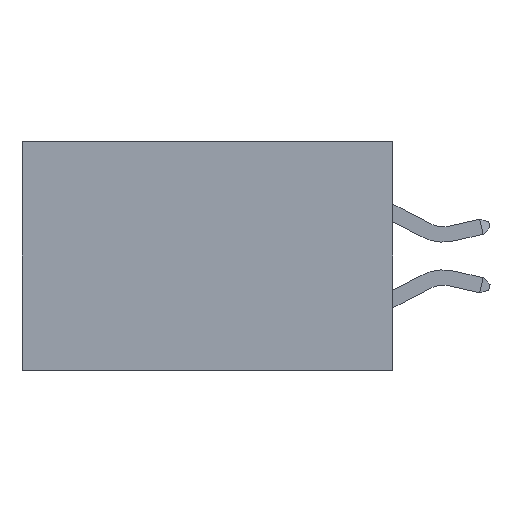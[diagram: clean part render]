
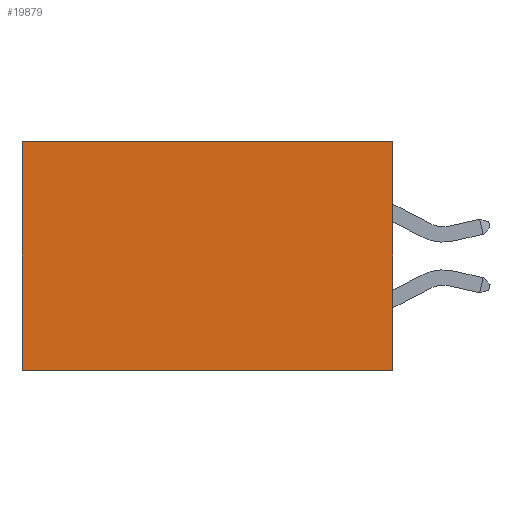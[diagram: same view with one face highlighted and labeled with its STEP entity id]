
A CAD part, left-side view. The second image highlights one B-rep face of the part: STEP entity #19879.
In plain terms, the highlighted planar face has unit normal (-1, 0, 0).
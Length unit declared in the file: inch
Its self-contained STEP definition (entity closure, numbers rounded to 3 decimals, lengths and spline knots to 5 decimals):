
#164 = DIRECTION ( 'NONE',  ( 0., 0., -1. ) ) ;
#1785 = CARTESIAN_POINT ( 'NONE',  ( 0.2875, 0., -0.37 ) ) ;
#3027 = CARTESIAN_POINT ( 'NONE',  ( 0.2875, 0.6, -0.37 ) ) ;
#3044 = CARTESIAN_POINT ( 'NONE',  ( 0.2875, 0., 0. ) ) ;
#3872 = LINE ( 'NONE', #5533, #8000 ) ;
#4692 = EDGE_CURVE ( 'NONE', #20896, #7798, #12696, .T. ) ;
#5347 = ORIENTED_EDGE ( 'NONE', *, *, #21614, .F. ) ;
#5533 = CARTESIAN_POINT ( 'NONE',  ( 0.2875, 0., 0. ) ) ;
#5863 = CARTESIAN_POINT ( 'NONE',  ( 0.2875, 0.6, 0. ) ) ;
#6748 = CARTESIAN_POINT ( 'NONE',  ( 0.2875, 0.6, 0. ) ) ;
#6987 = AXIS2_PLACEMENT_3D ( 'NONE', #3044, #8350, #20275 ) ;
#7798 = VERTEX_POINT ( 'NONE', #5863 ) ;
#8000 = VECTOR ( 'NONE', #164, 39.37008 ) ;
#8153 = CARTESIAN_POINT ( 'NONE',  ( 0.2875, 0., 0. ) ) ;
#8350 = DIRECTION ( 'NONE',  ( 1., 0., 0. ) ) ;
#8469 = DIRECTION ( 'NONE',  ( 0., 0., -1. ) ) ;
#9036 = EDGE_CURVE ( 'NONE', #7798, #14553, #19219, .T. ) ;
#9578 = VECTOR ( 'NONE', #21805, 39.37008 ) ;
#11141 = ORIENTED_EDGE ( 'NONE', *, *, #9036, .T. ) ;
#11676 = CARTESIAN_POINT ( 'NONE',  ( 0.2875, 0., -0.37 ) ) ;
#12696 = LINE ( 'NONE', #16119, #21182 ) ;
#14129 = LINE ( 'NONE', #11676, #9578 ) ;
#14167 = VECTOR ( 'NONE', #8469, 39.37008 ) ;
#14245 = VERTEX_POINT ( 'NONE', #1785 ) ;
#14553 = VERTEX_POINT ( 'NONE', #3027 ) ;
#16114 = FACE_OUTER_BOUND ( 'NONE', #18977, .T. ) ;
#16119 = CARTESIAN_POINT ( 'NONE',  ( 0.2875, 0., 0. ) ) ;
#17276 = ORIENTED_EDGE ( 'NONE', *, *, #21909, .F. ) ;
#18164 = ORIENTED_EDGE ( 'NONE', *, *, #4692, .T. ) ;
#18584 = PLANE ( 'NONE',  #6987 ) ;
#18977 = EDGE_LOOP ( 'NONE', ( #11141, #5347, #17276, #18164 ) ) ;
#19219 = LINE ( 'NONE', #6748, #14167 ) ;
#19456 = DIRECTION ( 'NONE',  ( 0., 1., 0. ) ) ;
#19879 = ADVANCED_FACE ( 'NONE', ( #16114 ), #18584, .F. ) ;
#20275 = DIRECTION ( 'NONE',  ( 0., 0., -1. ) ) ;
#20896 = VERTEX_POINT ( 'NONE', #8153 ) ;
#21182 = VECTOR ( 'NONE', #19456, 39.37008 ) ;
#21614 = EDGE_CURVE ( 'NONE', #14245, #14553, #14129, .T. ) ;
#21805 = DIRECTION ( 'NONE',  ( 0., 1., 0. ) ) ;
#21909 = EDGE_CURVE ( 'NONE', #20896, #14245, #3872, .T. ) ;
